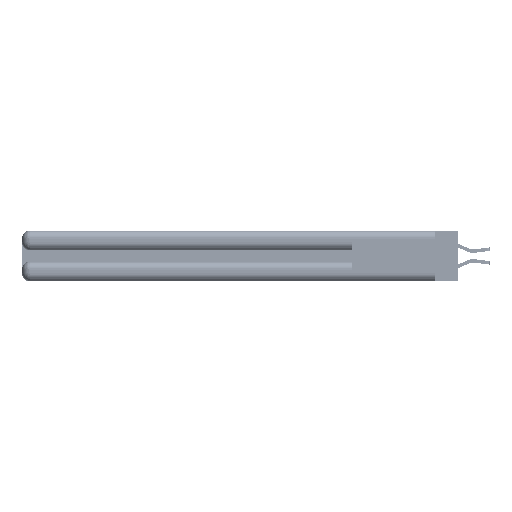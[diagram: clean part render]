
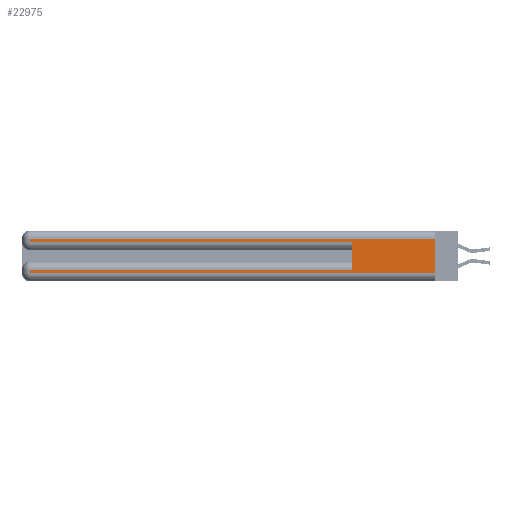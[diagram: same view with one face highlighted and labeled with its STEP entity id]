
A CAD part, left-side view. The second image highlights one B-rep face of the part: STEP entity #22975.
In plain terms, the highlighted planar face has unit normal (-1, 0, 0).
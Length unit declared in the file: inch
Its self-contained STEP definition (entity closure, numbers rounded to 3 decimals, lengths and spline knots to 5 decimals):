
#137 = ORIENTED_EDGE ( 'NONE', *, *, #20150, .F. ) ;
#851 = CARTESIAN_POINT ( 'NONE',  ( 0., 0., 0.085 ) ) ;
#3527 = CARTESIAN_POINT ( 'NONE',  ( 0., 0., 0.31 ) ) ;
#3562 = LINE ( 'NONE', #10824, #10101 ) ;
#4338 = ORIENTED_EDGE ( 'NONE', *, *, #32770, .T. ) ;
#4426 = EDGE_LOOP ( 'NONE', ( #137, #37045, #25308, #8964, #18218, #42838, #19191, #4338 ) ) ;
#4502 = LINE ( 'NONE', #40610, #25941 ) ;
#4699 = DIRECTION ( 'NONE',  ( 0., 1., 0. ) ) ;
#4792 = VECTOR ( 'NONE', #16206, 39.37008 ) ;
#6373 = VECTOR ( 'NONE', #24724, 39.37008 ) ;
#6493 = CARTESIAN_POINT ( 'NONE',  ( 0., 2.94, 0.37 ) ) ;
#6962 = VECTOR ( 'NONE', #33177, 39.37008 ) ;
#8964 = ORIENTED_EDGE ( 'NONE', *, *, #48167, .T. ) ;
#10101 = VECTOR ( 'NONE', #48637, 39.37008 ) ;
#10824 = CARTESIAN_POINT ( 'NONE',  ( 0., 0., 0.285 ) ) ;
#11834 = PLANE ( 'NONE',  #37484 ) ;
#16206 = DIRECTION ( 'NONE',  ( 0., 0., 1. ) ) ;
#18120 = CARTESIAN_POINT ( 'NONE',  ( 0., 2.94, 0.085 ) ) ;
#18218 = ORIENTED_EDGE ( 'NONE', *, *, #35900, .F. ) ;
#18473 = CARTESIAN_POINT ( 'NONE',  ( 0., 0., 0.31 ) ) ;
#18516 = VERTEX_POINT ( 'NONE', #42592 ) ;
#19191 = ORIENTED_EDGE ( 'NONE', *, *, #41459, .T. ) ;
#19567 = DIRECTION ( 'NONE',  ( 1., 0., 0. ) ) ;
#20021 = CARTESIAN_POINT ( 'NONE',  ( 0., 0., 0.06 ) ) ;
#20150 = EDGE_CURVE ( 'NONE', #46647, #31796, #4502, .T. ) ;
#20583 = VERTEX_POINT ( 'NONE', #43591 ) ;
#20941 = CARTESIAN_POINT ( 'NONE',  ( 0., 2.94, 0.37 ) ) ;
#22975 = ADVANCED_FACE ( 'NONE', ( #28931 ), #11834, .F. ) ;
#23809 = DIRECTION ( 'NONE',  ( 0., -1., 0. ) ) ;
#24045 = LINE ( 'NONE', #851, #42855 ) ;
#24724 = DIRECTION ( 'NONE',  ( 0., 0., -1. ) ) ;
#25308 = ORIENTED_EDGE ( 'NONE', *, *, #42402, .T. ) ;
#25941 = VECTOR ( 'NONE', #33079, 39.37008 ) ;
#26189 = VECTOR ( 'NONE', #26320, 39.37008 ) ;
#26227 = LINE ( 'NONE', #42608, #4792 ) ;
#26320 = DIRECTION ( 'NONE',  ( 0., 1., 0. ) ) ;
#26969 = CARTESIAN_POINT ( 'NONE',  ( 0., 0., 0.37 ) ) ;
#27351 = LINE ( 'NONE', #3527, #26189 ) ;
#28931 = FACE_OUTER_BOUND ( 'NONE', #4426, .T. ) ;
#30891 = VERTEX_POINT ( 'NONE', #44568 ) ;
#30954 = EDGE_CURVE ( 'NONE', #46647, #18516, #27351, .T. ) ;
#31796 = VERTEX_POINT ( 'NONE', #42664 ) ;
#32770 = EDGE_CURVE ( 'NONE', #30891, #31796, #48343, .T. ) ;
#33079 = DIRECTION ( 'NONE',  ( 0., 0., -1. ) ) ;
#33177 = DIRECTION ( 'NONE',  ( 0., 0., -1. ) ) ;
#33189 = VERTEX_POINT ( 'NONE', #48599 ) ;
#34136 = EDGE_CURVE ( 'NONE', #34227, #44641, #24045, .T. ) ;
#34227 = VERTEX_POINT ( 'NONE', #46683 ) ;
#35900 = EDGE_CURVE ( 'NONE', #34227, #33189, #26227, .T. ) ;
#35942 = VECTOR ( 'NONE', #23809, 39.37008 ) ;
#36583 = LINE ( 'NONE', #20941, #6373 ) ;
#37045 = ORIENTED_EDGE ( 'NONE', *, *, #30954, .T. ) ;
#37484 = AXIS2_PLACEMENT_3D ( 'NONE', #26969, #19567, #45871 ) ;
#38326 = LINE ( 'NONE', #6493, #6962 ) ;
#40610 = CARTESIAN_POINT ( 'NONE',  ( 0., 0., 0.37 ) ) ;
#41459 = EDGE_CURVE ( 'NONE', #44641, #30891, #36583, .T. ) ;
#42402 = EDGE_CURVE ( 'NONE', #18516, #20583, #38326, .T. ) ;
#42592 = CARTESIAN_POINT ( 'NONE',  ( 0., 2.94, 0.31 ) ) ;
#42608 = CARTESIAN_POINT ( 'NONE',  ( 0., 0.6, 0.145 ) ) ;
#42664 = CARTESIAN_POINT ( 'NONE',  ( 0., 0., 0.06 ) ) ;
#42838 = ORIENTED_EDGE ( 'NONE', *, *, #34136, .T. ) ;
#42855 = VECTOR ( 'NONE', #4699, 39.37008 ) ;
#43591 = CARTESIAN_POINT ( 'NONE',  ( 0., 2.94, 0.285 ) ) ;
#44568 = CARTESIAN_POINT ( 'NONE',  ( 0., 2.94, 0.06 ) ) ;
#44641 = VERTEX_POINT ( 'NONE', #18120 ) ;
#45871 = DIRECTION ( 'NONE',  ( 0., 0., -1. ) ) ;
#46647 = VERTEX_POINT ( 'NONE', #18473 ) ;
#46683 = CARTESIAN_POINT ( 'NONE',  ( 0., 0.6, 0.085 ) ) ;
#48167 = EDGE_CURVE ( 'NONE', #20583, #33189, #3562, .T. ) ;
#48343 = LINE ( 'NONE', #20021, #35942 ) ;
#48599 = CARTESIAN_POINT ( 'NONE',  ( 0., 0.6, 0.285 ) ) ;
#48637 = DIRECTION ( 'NONE',  ( 0., -1., 0. ) ) ;
